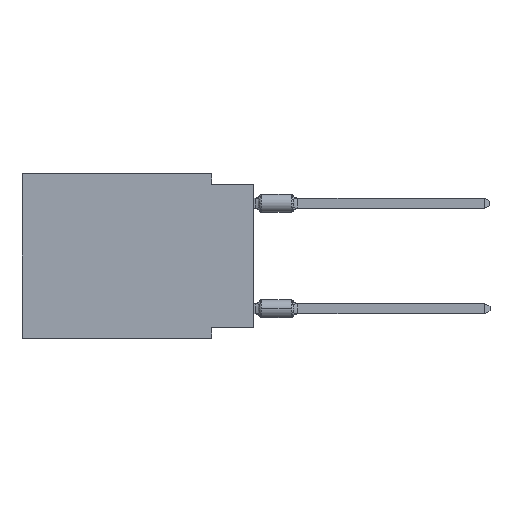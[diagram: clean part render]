
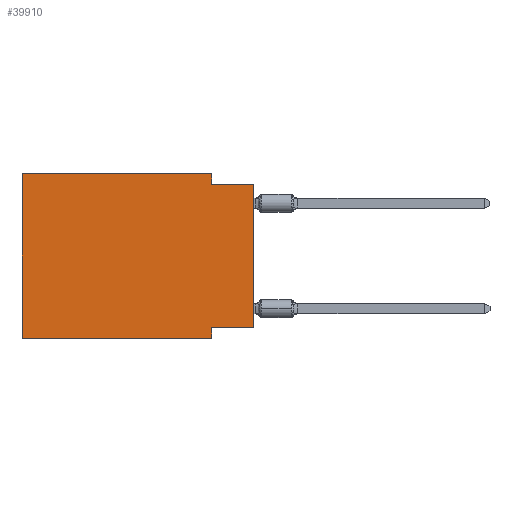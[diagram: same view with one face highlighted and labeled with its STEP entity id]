
A CAD part, left-side view. The second image highlights one B-rep face of the part: STEP entity #39910.
In plain terms, the highlighted planar face has unit normal (-1, 0, 0).
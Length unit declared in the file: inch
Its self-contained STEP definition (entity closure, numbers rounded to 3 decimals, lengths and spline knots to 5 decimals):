
#2776 = CARTESIAN_POINT ( 'NONE',  ( 0., 0.55, 0. ) ) ;
#3224 = VECTOR ( 'NONE', #26216, 39.37008 ) ;
#4130 = CARTESIAN_POINT ( 'NONE',  ( 0., 0.55, 0. ) ) ;
#8589 = DIRECTION ( 'NONE',  ( 0., -1., 0. ) ) ;
#8613 = EDGE_LOOP ( 'NONE', ( #29983, #29805, #43014, #8822, #38380, #31590, #45177, #42662 ) ) ;
#8822 = ORIENTED_EDGE ( 'NONE', *, *, #31856, .F. ) ;
#9599 = CARTESIAN_POINT ( 'NONE',  ( 0., 0., 0. ) ) ;
#9930 = LINE ( 'NONE', #14368, #31021 ) ;
#10267 = DIRECTION ( 'NONE',  ( 0., 0., -1. ) ) ;
#10435 = VERTEX_POINT ( 'NONE', #32368 ) ;
#11148 = FACE_OUTER_BOUND ( 'NONE', #8613, .T. ) ;
#11647 = EDGE_CURVE ( 'NONE', #24806, #42824, #35396, .T. ) ;
#13852 = VECTOR ( 'NONE', #33537, 39.37008 ) ;
#14368 = CARTESIAN_POINT ( 'NONE',  ( 0., 0.55, -0.39 ) ) ;
#14453 = CARTESIAN_POINT ( 'NONE',  ( 0., 0.55, -0.39 ) ) ;
#15287 = CARTESIAN_POINT ( 'NONE',  ( 0., 0.1, 0. ) ) ;
#15736 = CARTESIAN_POINT ( 'NONE',  ( 0., 0.1, -0.025 ) ) ;
#15882 = VERTEX_POINT ( 'NONE', #50031 ) ;
#16552 = LINE ( 'NONE', #51601, #13852 ) ;
#17591 = CARTESIAN_POINT ( 'NONE',  ( 0., 0.55, 0. ) ) ;
#18801 = VECTOR ( 'NONE', #8589, 39.37008 ) ;
#18862 = LINE ( 'NONE', #48908, #30107 ) ;
#19926 = EDGE_CURVE ( 'NONE', #39658, #22924, #24583, .T. ) ;
#20518 = EDGE_CURVE ( 'NONE', #29112, #39658, #31983, .T. ) ;
#22111 = DIRECTION ( 'NONE',  ( 0., 0., 1. ) ) ;
#22853 = EDGE_CURVE ( 'NONE', #15882, #10435, #16552, .T. ) ;
#22924 = VERTEX_POINT ( 'NONE', #32575 ) ;
#23779 = EDGE_CURVE ( 'NONE', #15882, #22924, #34912, .T. ) ;
#24572 = VECTOR ( 'NONE', #22111, 39.37008 ) ;
#24583 = LINE ( 'NONE', #47386, #29644 ) ;
#24806 = VERTEX_POINT ( 'NONE', #14453 ) ;
#25318 = CARTESIAN_POINT ( 'NONE',  ( 0., 0.1, 0. ) ) ;
#26216 = DIRECTION ( 'NONE',  ( 0., 0., 1. ) ) ;
#28003 = EDGE_CURVE ( 'NONE', #24806, #31998, #9930, .T. ) ;
#29112 = VERTEX_POINT ( 'NONE', #25318 ) ;
#29644 = VECTOR ( 'NONE', #47106, 39.37008 ) ;
#29678 = VECTOR ( 'NONE', #44788, 39.37008 ) ;
#29805 = ORIENTED_EDGE ( 'NONE', *, *, #19926, .F. ) ;
#29983 = ORIENTED_EDGE ( 'NONE', *, *, #23779, .T. ) ;
#30107 = VECTOR ( 'NONE', #10267, 39.37008 ) ;
#31021 = VECTOR ( 'NONE', #44678, 39.37008 ) ;
#31590 = ORIENTED_EDGE ( 'NONE', *, *, #28003, .T. ) ;
#31856 = EDGE_CURVE ( 'NONE', #42824, #29112, #42242, .T. ) ;
#31983 = LINE ( 'NONE', #15287, #29678 ) ;
#31998 = VERTEX_POINT ( 'NONE', #34727 ) ;
#32368 = CARTESIAN_POINT ( 'NONE',  ( 0., 0.1, -0.365 ) ) ;
#32575 = CARTESIAN_POINT ( 'NONE',  ( 0., 0., -0.025 ) ) ;
#33537 = DIRECTION ( 'NONE',  ( 0., 1., 0. ) ) ;
#34727 = CARTESIAN_POINT ( 'NONE',  ( 0., 0.1, -0.39 ) ) ;
#34912 = LINE ( 'NONE', #9599, #24572 ) ;
#35396 = LINE ( 'NONE', #17591, #3224 ) ;
#36186 = PLANE ( 'NONE',  #36912 ) ;
#36912 = AXIS2_PLACEMENT_3D ( 'NONE', #2776, #52150, #49252 ) ;
#38380 = ORIENTED_EDGE ( 'NONE', *, *, #11647, .F. ) ;
#39658 = VERTEX_POINT ( 'NONE', #15736 ) ;
#39910 = ADVANCED_FACE ( 'NONE', ( #11148 ), #36186, .F. ) ;
#42242 = LINE ( 'NONE', #4130, #18801 ) ;
#42662 = ORIENTED_EDGE ( 'NONE', *, *, #22853, .F. ) ;
#42824 = VERTEX_POINT ( 'NONE', #43203 ) ;
#43014 = ORIENTED_EDGE ( 'NONE', *, *, #20518, .F. ) ;
#43203 = CARTESIAN_POINT ( 'NONE',  ( 0., 0.55, 0. ) ) ;
#44678 = DIRECTION ( 'NONE',  ( 0., -1., 0. ) ) ;
#44788 = DIRECTION ( 'NONE',  ( 0., 0., -1. ) ) ;
#45177 = ORIENTED_EDGE ( 'NONE', *, *, #46243, .F. ) ;
#46243 = EDGE_CURVE ( 'NONE', #10435, #31998, #18862, .T. ) ;
#47106 = DIRECTION ( 'NONE',  ( 0., -1., 0. ) ) ;
#47386 = CARTESIAN_POINT ( 'NONE',  ( 0., 0., -0.025 ) ) ;
#48908 = CARTESIAN_POINT ( 'NONE',  ( 0., 0.1, -0.39 ) ) ;
#49252 = DIRECTION ( 'NONE',  ( 0., 0., -1. ) ) ;
#50031 = CARTESIAN_POINT ( 'NONE',  ( 0., 0., -0.365 ) ) ;
#51601 = CARTESIAN_POINT ( 'NONE',  ( 0., 0., -0.365 ) ) ;
#52150 = DIRECTION ( 'NONE',  ( 1., 0., 0. ) ) ;
